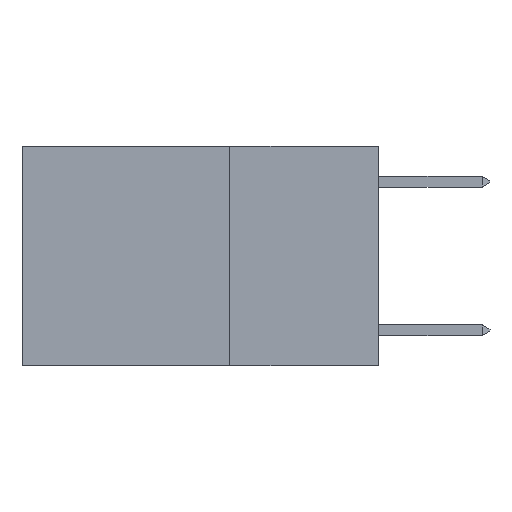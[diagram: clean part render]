
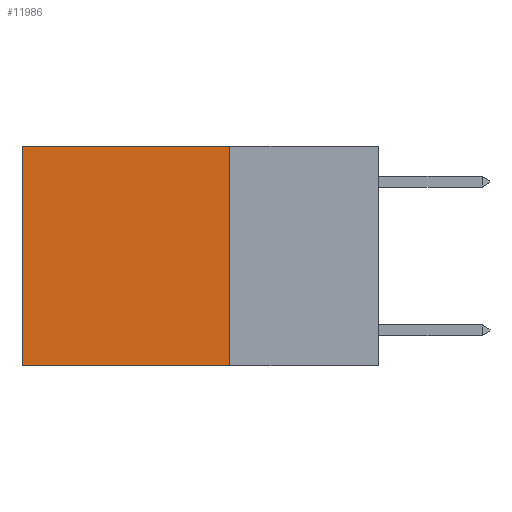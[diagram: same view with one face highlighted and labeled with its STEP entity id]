
A CAD part, left-side view. The second image highlights one B-rep face of the part: STEP entity #11986.
In plain terms, the highlighted planar face has unit normal (-1, 0, 0).
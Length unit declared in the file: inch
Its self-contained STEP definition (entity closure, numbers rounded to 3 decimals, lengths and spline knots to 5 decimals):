
#53 = EDGE_CURVE ( 'NONE', #8850, #11132, #9641, .T. ) ;
#186 = FACE_OUTER_BOUND ( 'NONE', #7566, .T. ) ;
#654 = VERTEX_POINT ( 'NONE', #6919 ) ;
#1546 = EDGE_CURVE ( 'NONE', #654, #11132, #11174, .T. ) ;
#1654 = CARTESIAN_POINT ( 'NONE',  ( 0.2625, 0.25, 0. ) ) ;
#1846 = LINE ( 'NONE', #7453, #4265 ) ;
#2149 = CARTESIAN_POINT ( 'NONE',  ( 0.2625, 0.25, 0. ) ) ;
#2265 = VECTOR ( 'NONE', #2673, 39.37008 ) ;
#2638 = EDGE_CURVE ( 'NONE', #3278, #654, #1846, .T. ) ;
#2673 = DIRECTION ( 'NONE',  ( 0., 0., -1. ) ) ;
#2833 = DIRECTION ( 'NONE',  ( 0., 0., -1. ) ) ;
#3062 = DIRECTION ( 'NONE',  ( 1., 0., 0. ) ) ;
#3278 = VERTEX_POINT ( 'NONE', #1654 ) ;
#3747 = ORIENTED_EDGE ( 'NONE', *, *, #1546, .T. ) ;
#3915 = PLANE ( 'NONE',  #5315 ) ;
#4265 = VECTOR ( 'NONE', #11011, 39.37008 ) ;
#4544 = CARTESIAN_POINT ( 'NONE',  ( 0.2625, 0.6, 0. ) ) ;
#4887 = ORIENTED_EDGE ( 'NONE', *, *, #53, .F. ) ;
#4903 = VECTOR ( 'NONE', #6853, 39.37008 ) ;
#5315 = AXIS2_PLACEMENT_3D ( 'NONE', #2149, #3062, #9626 ) ;
#5385 = CARTESIAN_POINT ( 'NONE',  ( 0.2625, 0.25, -0.37 ) ) ;
#6853 = DIRECTION ( 'NONE',  ( 0., 1., 0. ) ) ;
#6919 = CARTESIAN_POINT ( 'NONE',  ( 0.2625, 0.6, 0. ) ) ;
#7270 = LINE ( 'NONE', #10143, #2265 ) ;
#7453 = CARTESIAN_POINT ( 'NONE',  ( 0.2625, 0.25, 0. ) ) ;
#7566 = EDGE_LOOP ( 'NONE', ( #3747, #4887, #10112, #11869 ) ) ;
#8780 = VECTOR ( 'NONE', #2833, 39.37008 ) ;
#8850 = VERTEX_POINT ( 'NONE', #5385 ) ;
#9626 = DIRECTION ( 'NONE',  ( 0., 0., -1. ) ) ;
#9641 = LINE ( 'NONE', #10568, #4903 ) ;
#10112 = ORIENTED_EDGE ( 'NONE', *, *, #11676, .F. ) ;
#10143 = CARTESIAN_POINT ( 'NONE',  ( 0.2625, 0.25, 0. ) ) ;
#10568 = CARTESIAN_POINT ( 'NONE',  ( 0.2625, 0.25, -0.37 ) ) ;
#11011 = DIRECTION ( 'NONE',  ( 0., 1., 0. ) ) ;
#11132 = VERTEX_POINT ( 'NONE', #11135 ) ;
#11135 = CARTESIAN_POINT ( 'NONE',  ( 0.2625, 0.6, -0.37 ) ) ;
#11174 = LINE ( 'NONE', #4544, #8780 ) ;
#11676 = EDGE_CURVE ( 'NONE', #3278, #8850, #7270, .T. ) ;
#11869 = ORIENTED_EDGE ( 'NONE', *, *, #2638, .T. ) ;
#11986 = ADVANCED_FACE ( 'NONE', ( #186 ), #3915, .F. ) ;
